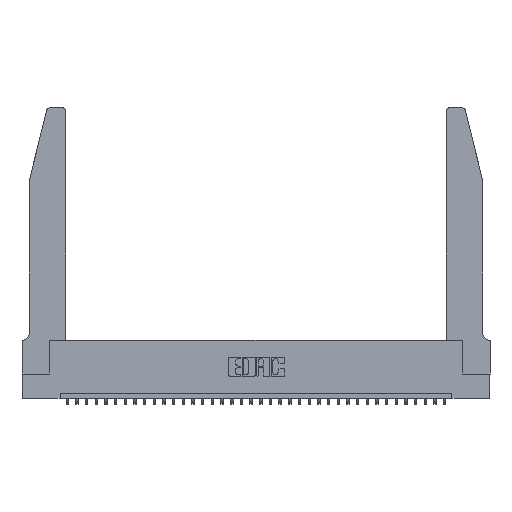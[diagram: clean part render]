
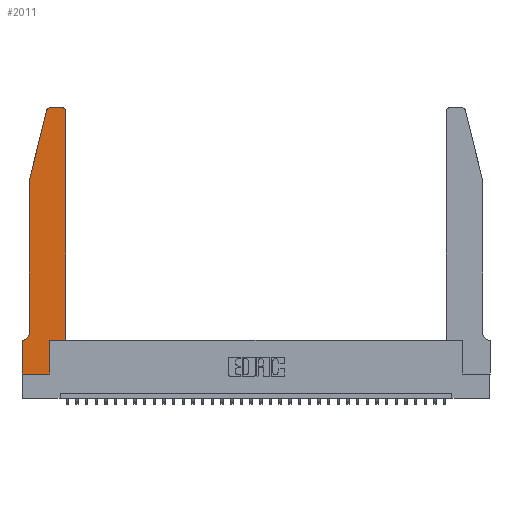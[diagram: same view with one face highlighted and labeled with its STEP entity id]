
A CAD part, top view. The second image highlights one B-rep face of the part: STEP entity #2011.
In plain terms, the highlighted planar face has unit normal (0, 0, 1).
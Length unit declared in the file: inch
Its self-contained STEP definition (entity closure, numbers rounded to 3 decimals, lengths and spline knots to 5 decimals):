
#78 = LINE ( 'NONE', #16329, #31118 ) ;
#171 = LINE ( 'NONE', #24873, #19796 ) ;
#286 = DIRECTION ( 'NONE',  ( 1., 0., 0. ) ) ;
#681 = ORIENTED_EDGE ( 'NONE', *, *, #9149, .T. ) ;
#1157 = VERTEX_POINT ( 'NONE', #2306 ) ;
#1410 = EDGE_CURVE ( 'NONE', #19073, #11192, #78, .T. ) ;
#2011 = ADVANCED_FACE ( 'NONE', ( #23874 ), #26581, .T. ) ;
#2306 = CARTESIAN_POINT ( 'NONE',  ( 0.4505, 0.35, 0.37 ) ) ;
#2356 = EDGE_CURVE ( 'NONE', #34949, #2368, #12812, .T. ) ;
#2368 = VERTEX_POINT ( 'NONE', #13479 ) ;
#2547 = VECTOR ( 'NONE', #26370, 39.37008 ) ;
#3205 = ORIENTED_EDGE ( 'NONE', *, *, #23972, .T. ) ;
#3499 = EDGE_CURVE ( 'NONE', #17963, #34949, #21618, .T. ) ;
#3589 = AXIS2_PLACEMENT_3D ( 'NONE', #7740, #15940, #10837 ) ;
#4256 = LINE ( 'NONE', #11089, #8472 ) ;
#5030 = VECTOR ( 'NONE', #7719, 39.37008 ) ;
#5535 = ORIENTED_EDGE ( 'NONE', *, *, #32851, .T. ) ;
#7430 = CARTESIAN_POINT ( 'NONE',  ( 0., 0., 0.37 ) ) ;
#7719 = DIRECTION ( 'NONE',  ( 0., -1., 0. ) ) ;
#7740 = CARTESIAN_POINT ( 'NONE',  ( 0.0055, 0.42, 0.37 ) ) ;
#8005 = DIRECTION ( 'NONE',  ( -1., 0., 0. ) ) ;
#8373 = DIRECTION ( 'NONE',  ( 0., 1., 0. ) ) ;
#8472 = VECTOR ( 'NONE', #32522, 39.37008 ) ;
#8480 = VECTOR ( 'NONE', #15705, 39.37008 ) ;
#8710 = ORIENTED_EDGE ( 'NONE', *, *, #15698, .T. ) ;
#9018 = CARTESIAN_POINT ( 'NONE',  ( 0.4205, 2.72, 0.37 ) ) ;
#9149 = EDGE_CURVE ( 'NONE', #1157, #10226, #16592, .T. ) ;
#10226 = VERTEX_POINT ( 'NONE', #29405 ) ;
#10690 = LINE ( 'NONE', #34089, #8480 ) ;
#10837 = DIRECTION ( 'NONE',  ( -1., 0., 0. ) ) ;
#11089 = CARTESIAN_POINT ( 'NONE',  ( 0.4505, 0.35, 0.37 ) ) ;
#11192 = VERTEX_POINT ( 'NONE', #14954 ) ;
#11659 = ORIENTED_EDGE ( 'NONE', *, *, #22165, .T. ) ;
#11886 = ORIENTED_EDGE ( 'NONE', *, *, #22757, .T. ) ;
#12097 = CIRCLE ( 'NONE', #32508, 0.03 ) ;
#12812 = LINE ( 'NONE', #13704, #19602 ) ;
#13183 = VERTEX_POINT ( 'NONE', #20787 ) ;
#13250 = DIRECTION ( 'NONE',  ( 1., 0., 0. ) ) ;
#13479 = CARTESIAN_POINT ( 'NONE',  ( 0.2865, 0.35, 0.37 ) ) ;
#13704 = CARTESIAN_POINT ( 'NONE',  ( 0.2865, 0.35, 0.37 ) ) ;
#14396 = VECTOR ( 'NONE', #13250, 39.37008 ) ;
#14954 = CARTESIAN_POINT ( 'NONE',  ( 0.0755, 2., 0.37 ) ) ;
#15698 = EDGE_CURVE ( 'NONE', #22431, #19073, #12097, .T. ) ;
#15705 = DIRECTION ( 'NONE',  ( 0., -1., 0. ) ) ;
#15940 = DIRECTION ( 'NONE',  ( 0., 0., -1. ) ) ;
#16329 = CARTESIAN_POINT ( 'NONE',  ( 0.0755, 2., 0.37 ) ) ;
#16592 = LINE ( 'NONE', #34236, #2547 ) ;
#17726 = AXIS2_PLACEMENT_3D ( 'NONE', #9018, #20189, #25616 ) ;
#17963 = VERTEX_POINT ( 'NONE', #7430 ) ;
#18652 = CARTESIAN_POINT ( 'NONE',  ( 0., 0., 0.37 ) ) ;
#19073 = VERTEX_POINT ( 'NONE', #25598 ) ;
#19118 = CARTESIAN_POINT ( 'NONE',  ( 0.284, 2.75, 0.37 ) ) ;
#19363 = AXIS2_PLACEMENT_3D ( 'NONE', #34804, #32162, #286 ) ;
#19602 = VECTOR ( 'NONE', #8373, 39.37008 ) ;
#19796 = VECTOR ( 'NONE', #32924, 39.37008 ) ;
#19971 = DIRECTION ( 'NONE',  ( 1., 0., 0. ) ) ;
#20186 = VERTEX_POINT ( 'NONE', #22297 ) ;
#20189 = DIRECTION ( 'NONE',  ( 0., 0., 1. ) ) ;
#20787 = CARTESIAN_POINT ( 'NONE',  ( 0., 0.35, 0.37 ) ) ;
#21618 = LINE ( 'NONE', #26645, #14396 ) ;
#22165 = EDGE_CURVE ( 'NONE', #11192, #32459, #10690, .T. ) ;
#22297 = CARTESIAN_POINT ( 'NONE',  ( 0.4205, 2.75, 0.37 ) ) ;
#22431 = VERTEX_POINT ( 'NONE', #19118 ) ;
#22757 = EDGE_CURVE ( 'NONE', #10226, #20186, #32647, .T. ) ;
#23676 = CIRCLE ( 'NONE', #3589, 0.07 ) ;
#23874 = FACE_OUTER_BOUND ( 'NONE', #30632, .T. ) ;
#23972 = EDGE_CURVE ( 'NONE', #32459, #31945, #23676, .T. ) ;
#24441 = EDGE_CURVE ( 'NONE', #20186, #22431, #30323, .T. ) ;
#24690 = EDGE_CURVE ( 'NONE', #31945, #13183, #171, .T. ) ;
#24873 = CARTESIAN_POINT ( 'NONE',  ( 0.0755, 0.35, 0.37 ) ) ;
#25031 = ORIENTED_EDGE ( 'NONE', *, *, #1410, .T. ) ;
#25127 = CARTESIAN_POINT ( 'NONE',  ( 0.284, 2.72, 0.37 ) ) ;
#25598 = CARTESIAN_POINT ( 'NONE',  ( 0.25487, 2.72718, 0.37 ) ) ;
#25616 = DIRECTION ( 'NONE',  ( 1., 0., 0. ) ) ;
#26370 = DIRECTION ( 'NONE',  ( 0., 1., 0. ) ) ;
#26581 = PLANE ( 'NONE',  #19363 ) ;
#26607 = CARTESIAN_POINT ( 'NONE',  ( 0.2605, 2.75, 0.37 ) ) ;
#26645 = CARTESIAN_POINT ( 'NONE',  ( 0., 0., 0.37 ) ) ;
#28857 = ORIENTED_EDGE ( 'NONE', *, *, #24441, .T. ) ;
#29405 = CARTESIAN_POINT ( 'NONE',  ( 0.4505, 2.72, 0.37 ) ) ;
#30124 = DIRECTION ( 'NONE',  ( -0.239, -0.971, 0. ) ) ;
#30323 = LINE ( 'NONE', #26607, #31682 ) ;
#30445 = ORIENTED_EDGE ( 'NONE', *, *, #3499, .T. ) ;
#30632 = EDGE_LOOP ( 'NONE', ( #28857, #8710, #25031, #11659, #3205, #33003, #34616, #30445, #34831, #5535, #681, #11886 ) ) ;
#30801 = DIRECTION ( 'NONE',  ( 0., 0., 1. ) ) ;
#30917 = CARTESIAN_POINT ( 'NONE',  ( 0.0055, 0.35, 0.37 ) ) ;
#31118 = VECTOR ( 'NONE', #30124, 39.37008 ) ;
#31682 = VECTOR ( 'NONE', #8005, 39.37008 ) ;
#31945 = VERTEX_POINT ( 'NONE', #30917 ) ;
#32162 = DIRECTION ( 'NONE',  ( 0., 0., 1. ) ) ;
#32459 = VERTEX_POINT ( 'NONE', #33885 ) ;
#32508 = AXIS2_PLACEMENT_3D ( 'NONE', #25127, #30801, #19971 ) ;
#32522 = DIRECTION ( 'NONE',  ( 1., 0., 0. ) ) ;
#32647 = CIRCLE ( 'NONE', #17726, 0.03 ) ;
#32851 = EDGE_CURVE ( 'NONE', #2368, #1157, #4256, .T. ) ;
#32924 = DIRECTION ( 'NONE',  ( -1., 0., 0. ) ) ;
#33003 = ORIENTED_EDGE ( 'NONE', *, *, #24690, .T. ) ;
#33600 = EDGE_CURVE ( 'NONE', #13183, #17963, #34335, .T. ) ;
#33885 = CARTESIAN_POINT ( 'NONE',  ( 0.0755, 0.42, 0.37 ) ) ;
#34089 = CARTESIAN_POINT ( 'NONE',  ( 0.0755, 2., 0.37 ) ) ;
#34188 = CARTESIAN_POINT ( 'NONE',  ( 0.2865, 0., 0.37 ) ) ;
#34236 = CARTESIAN_POINT ( 'NONE',  ( 0.4505, 0.35, 0.37 ) ) ;
#34335 = LINE ( 'NONE', #18652, #5030 ) ;
#34616 = ORIENTED_EDGE ( 'NONE', *, *, #33600, .T. ) ;
#34804 = CARTESIAN_POINT ( 'NONE',  ( 0., 0.35, 0.37 ) ) ;
#34831 = ORIENTED_EDGE ( 'NONE', *, *, #2356, .T. ) ;
#34949 = VERTEX_POINT ( 'NONE', #34188 ) ;
